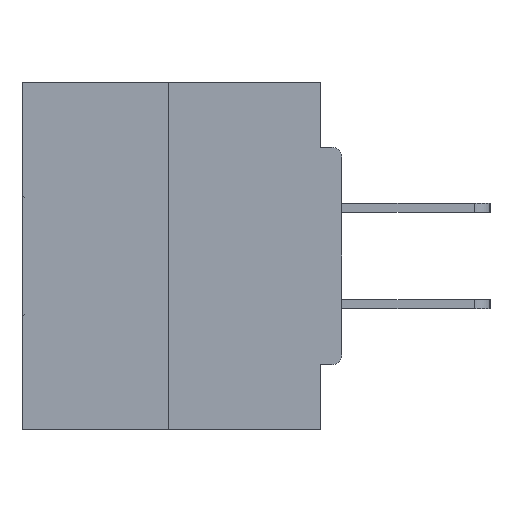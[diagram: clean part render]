
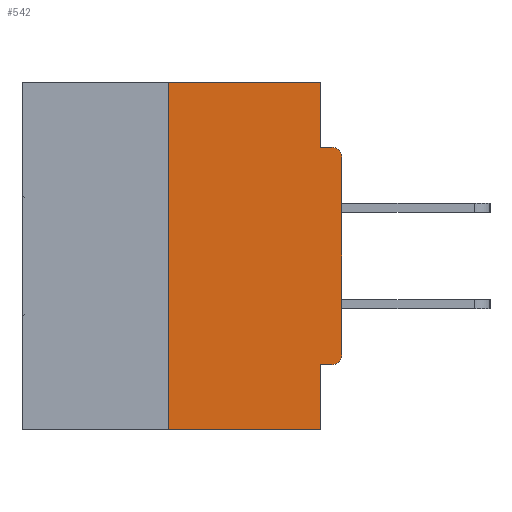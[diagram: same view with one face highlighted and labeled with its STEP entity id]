
A CAD part, left-side view. The second image highlights one B-rep face of the part: STEP entity #542.
In plain terms, the highlighted planar face has unit normal (-1, 0, 0).
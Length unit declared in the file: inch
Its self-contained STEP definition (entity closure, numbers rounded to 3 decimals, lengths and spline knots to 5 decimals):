
#401 = LINE ( 'NONE', #23293, #32335 ) ;
#542 = ADVANCED_FACE ( 'NONE', ( #5020 ), #17921, .F. ) ;
#558 = ORIENTED_EDGE ( 'NONE', *, *, #39031, .T. ) ;
#1082 = EDGE_CURVE ( 'NONE', #15308, #36031, #21844, .T. ) ;
#1291 = DIRECTION ( 'NONE',  ( 0., 1., 0. ) ) ;
#1403 = DIRECTION ( 'NONE',  ( -1., 0., 0. ) ) ;
#1707 = DIRECTION ( 'NONE',  ( 0., 0., 1. ) ) ;
#1912 = LINE ( 'NONE', #11832, #33773 ) ;
#1925 = DIRECTION ( 'NONE',  ( 0., -1., 0. ) ) ;
#2209 = AXIS2_PLACEMENT_3D ( 'NONE', #30510, #1403, #4583 ) ;
#2737 = EDGE_CURVE ( 'NONE', #28972, #40315, #5458, .T. ) ;
#2749 = CARTESIAN_POINT ( 'NONE',  ( 0., 0.015, -0.3915 ) ) ;
#3107 = VECTOR ( 'NONE', #9241, 39.37008 ) ;
#3216 = ORIENTED_EDGE ( 'NONE', *, *, #13405, .T. ) ;
#3304 = ORIENTED_EDGE ( 'NONE', *, *, #36648, .T. ) ;
#4508 = CARTESIAN_POINT ( 'NONE',  ( 0., 0., -0.3915 ) ) ;
#4583 = DIRECTION ( 'NONE',  ( 0., 0., -1. ) ) ;
#4845 = VECTOR ( 'NONE', #23982, 39.37008 ) ;
#4930 = CARTESIAN_POINT ( 'NONE',  ( 0., 0.031, -0.5 ) ) ;
#5020 = FACE_OUTER_BOUND ( 'NONE', #5901, .T. ) ;
#5160 = CARTESIAN_POINT ( 'NONE',  ( 0., 0.25, -0.5 ) ) ;
#5458 = LINE ( 'NONE', #25185, #3107 ) ;
#5901 = EDGE_LOOP ( 'NONE', ( #37211, #11782, #3304, #25346, #19910, #558, #3216, #38486, #11545, #16729 ) ) ;
#6204 = CIRCLE ( 'NONE', #29988, 0.015 ) ;
#6207 = CARTESIAN_POINT ( 'NONE',  ( 0., 0.015, -0.4065 ) ) ;
#6567 = EDGE_CURVE ( 'NONE', #17395, #18377, #35426, .T. ) ;
#6690 = EDGE_CURVE ( 'NONE', #29601, #24620, #401, .T. ) ;
#8544 = VECTOR ( 'NONE', #35845, 39.37008 ) ;
#9241 = DIRECTION ( 'NONE',  ( 0., 0., -1. ) ) ;
#10736 = LINE ( 'NONE', #17098, #39648 ) ;
#10993 = CARTESIAN_POINT ( 'NONE',  ( 0., 0., -0.4065 ) ) ;
#11544 = DIRECTION ( 'NONE',  ( 0., 0., -1. ) ) ;
#11545 = ORIENTED_EDGE ( 'NONE', *, *, #17603, .F. ) ;
#11609 = LINE ( 'NONE', #37163, #4845 ) ;
#11782 = ORIENTED_EDGE ( 'NONE', *, *, #6690, .F. ) ;
#11832 = CARTESIAN_POINT ( 'NONE',  ( 0., 0., 0. ) ) ;
#12253 = LINE ( 'NONE', #41391, #29822 ) ;
#13405 = EDGE_CURVE ( 'NONE', #31172, #15308, #1912, .T. ) ;
#13547 = LINE ( 'NONE', #10993, #31394 ) ;
#13915 = DIRECTION ( 'NONE',  ( 0., -1., 0. ) ) ;
#15308 = VERTEX_POINT ( 'NONE', #26352 ) ;
#16729 = ORIENTED_EDGE ( 'NONE', *, *, #2737, .F. ) ;
#17098 = CARTESIAN_POINT ( 'NONE',  ( 0., 0.46, 0. ) ) ;
#17395 = VERTEX_POINT ( 'NONE', #31885 ) ;
#17603 = EDGE_CURVE ( 'NONE', #40315, #36031, #11609, .T. ) ;
#17921 = PLANE ( 'NONE',  #23409 ) ;
#18377 = VERTEX_POINT ( 'NONE', #4930 ) ;
#19910 = ORIENTED_EDGE ( 'NONE', *, *, #33910, .F. ) ;
#21223 = DIRECTION ( 'NONE',  ( 0., 0., -1. ) ) ;
#21670 = EDGE_CURVE ( 'NONE', #24620, #28972, #10736, .T. ) ;
#21844 = CIRCLE ( 'NONE', #2209, 0.015 ) ;
#23293 = CARTESIAN_POINT ( 'NONE',  ( 0., 0.25, 0. ) ) ;
#23409 = AXIS2_PLACEMENT_3D ( 'NONE', #30946, #40703, #11544 ) ;
#23982 = DIRECTION ( 'NONE',  ( 0., -1., 0. ) ) ;
#24438 = CARTESIAN_POINT ( 'NONE',  ( 0., 0.031, -0.0935 ) ) ;
#24620 = VERTEX_POINT ( 'NONE', #36078 ) ;
#25185 = CARTESIAN_POINT ( 'NONE',  ( 0., 0.031, 0. ) ) ;
#25346 = ORIENTED_EDGE ( 'NONE', *, *, #6567, .F. ) ;
#26352 = CARTESIAN_POINT ( 'NONE',  ( 0., 0., -0.1085 ) ) ;
#27029 = CARTESIAN_POINT ( 'NONE',  ( 0., 0.015, -0.0935 ) ) ;
#28657 = DIRECTION ( 'NONE',  ( -1., 0., 0. ) ) ;
#28972 = VERTEX_POINT ( 'NONE', #32258 ) ;
#29489 = DIRECTION ( 'NONE',  ( 0., 0., 1. ) ) ;
#29601 = VERTEX_POINT ( 'NONE', #5160 ) ;
#29822 = VECTOR ( 'NONE', #1925, 39.37008 ) ;
#29988 = AXIS2_PLACEMENT_3D ( 'NONE', #2749, #28657, #21223 ) ;
#30510 = CARTESIAN_POINT ( 'NONE',  ( 0., 0.015, -0.1085 ) ) ;
#30946 = CARTESIAN_POINT ( 'NONE',  ( 0., 0.46, 0. ) ) ;
#31078 = VERTEX_POINT ( 'NONE', #6207 ) ;
#31172 = VERTEX_POINT ( 'NONE', #4508 ) ;
#31394 = VECTOR ( 'NONE', #1291, 39.37008 ) ;
#31885 = CARTESIAN_POINT ( 'NONE',  ( 0., 0.031, -0.4065 ) ) ;
#32258 = CARTESIAN_POINT ( 'NONE',  ( 0., 0.031, 0. ) ) ;
#32335 = VECTOR ( 'NONE', #29489, 39.37008 ) ;
#33773 = VECTOR ( 'NONE', #1707, 39.37008 ) ;
#33910 = EDGE_CURVE ( 'NONE', #31078, #17395, #13547, .T. ) ;
#35426 = LINE ( 'NONE', #35646, #8544 ) ;
#35646 = CARTESIAN_POINT ( 'NONE',  ( 0., 0.031, -0.5 ) ) ;
#35845 = DIRECTION ( 'NONE',  ( 0., 0., -1. ) ) ;
#36031 = VERTEX_POINT ( 'NONE', #27029 ) ;
#36078 = CARTESIAN_POINT ( 'NONE',  ( 0., 0.25, 0. ) ) ;
#36648 = EDGE_CURVE ( 'NONE', #29601, #18377, #12253, .T. ) ;
#37163 = CARTESIAN_POINT ( 'NONE',  ( 0., 0., -0.0935 ) ) ;
#37211 = ORIENTED_EDGE ( 'NONE', *, *, #21670, .F. ) ;
#38486 = ORIENTED_EDGE ( 'NONE', *, *, #1082, .T. ) ;
#39031 = EDGE_CURVE ( 'NONE', #31078, #31172, #6204, .T. ) ;
#39648 = VECTOR ( 'NONE', #13915, 39.37008 ) ;
#40315 = VERTEX_POINT ( 'NONE', #24438 ) ;
#40703 = DIRECTION ( 'NONE',  ( 1., 0., 0. ) ) ;
#41391 = CARTESIAN_POINT ( 'NONE',  ( 0., 0.46, -0.5 ) ) ;
